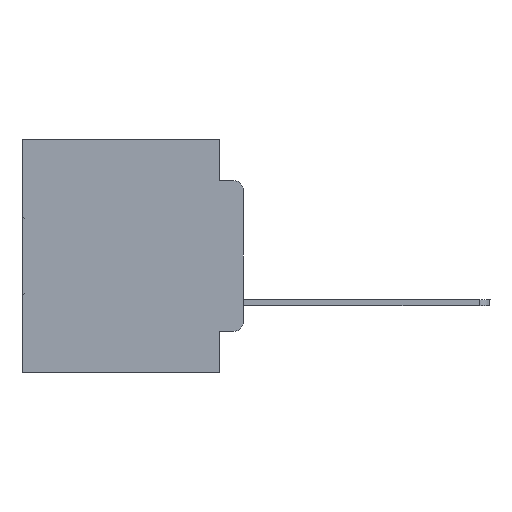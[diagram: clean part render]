
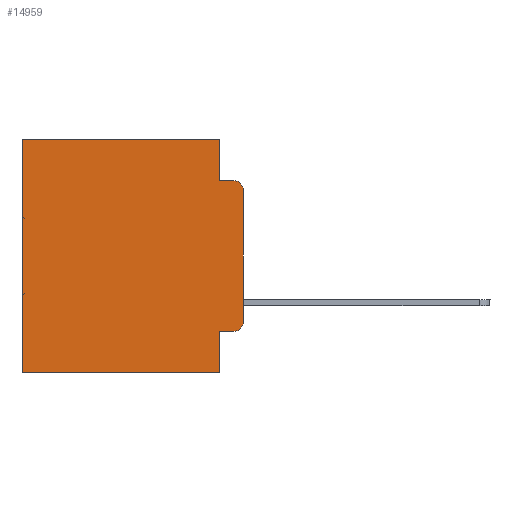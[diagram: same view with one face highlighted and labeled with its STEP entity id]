
A CAD part, left-side view. The second image highlights one B-rep face of the part: STEP entity #14959.
In plain terms, the highlighted planar face has unit normal (-1, 0, 0).
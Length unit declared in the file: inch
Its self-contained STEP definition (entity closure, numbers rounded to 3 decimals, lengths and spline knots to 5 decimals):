
#21 = DIRECTION ( 'NONE',  ( 0., 0., -1. ) ) ;
#1100 = VECTOR ( 'NONE', #27596, 39.37008 ) ;
#1137 = VECTOR ( 'NONE', #7769, 39.37008 ) ;
#1483 = ORIENTED_EDGE ( 'NONE', *, *, #3635, .T. ) ;
#2066 = CIRCLE ( 'NONE', #21026, 0.02 ) ;
#2542 = LINE ( 'NONE', #3341, #5845 ) ;
#3288 = VERTEX_POINT ( 'NONE', #8093 ) ;
#3341 = CARTESIAN_POINT ( 'NONE',  ( 0.298, 0., 0. ) ) ;
#3451 = DIRECTION ( 'NONE',  ( 0., 0., -1. ) ) ;
#3635 = EDGE_CURVE ( 'NONE', #31642, #13835, #26055, .T. ) ;
#4480 = ORIENTED_EDGE ( 'NONE', *, *, #25943, .T. ) ;
#4596 = CARTESIAN_POINT ( 'NONE',  ( 0.298, 0.02, -0.3915 ) ) ;
#4645 = EDGE_CURVE ( 'NONE', #8941, #17580, #16292, .T. ) ;
#5450 = VECTOR ( 'NONE', #10947, 39.37008 ) ;
#5484 = CIRCLE ( 'NONE', #14705, 0.02 ) ;
#5627 = LINE ( 'NONE', #23620, #17270 ) ;
#5845 = VECTOR ( 'NONE', #31802, 39.37008 ) ;
#5939 = VERTEX_POINT ( 'NONE', #24429 ) ;
#6153 = PLANE ( 'NONE',  #25862 ) ;
#6167 = VERTEX_POINT ( 'NONE', #28332 ) ;
#6237 = LINE ( 'NONE', #16592, #19477 ) ;
#7073 = CARTESIAN_POINT ( 'NONE',  ( 0.298, 0.051, -0.0885 ) ) ;
#7769 = DIRECTION ( 'NONE',  ( 0., -1., 0. ) ) ;
#7845 = DIRECTION ( 'NONE',  ( 0., 0., -1. ) ) ;
#7873 = ORIENTED_EDGE ( 'NONE', *, *, #23810, .F. ) ;
#8006 = LINE ( 'NONE', #10394, #9837 ) ;
#8093 = CARTESIAN_POINT ( 'NONE',  ( 0.298, 0.02, -0.4115 ) ) ;
#8941 = VERTEX_POINT ( 'NONE', #30897 ) ;
#9683 = ORIENTED_EDGE ( 'NONE', *, *, #16460, .F. ) ;
#9837 = VECTOR ( 'NONE', #7845, 39.37008 ) ;
#10394 = CARTESIAN_POINT ( 'NONE',  ( 0.298, 0.473, 0. ) ) ;
#10399 = DIRECTION ( 'NONE',  ( 0., 0., -1. ) ) ;
#10947 = DIRECTION ( 'NONE',  ( 0., 1., 0. ) ) ;
#12906 = DIRECTION ( 'NONE',  ( -1., 0., 0. ) ) ;
#13035 = ORIENTED_EDGE ( 'NONE', *, *, #18951, .T. ) ;
#13082 = VERTEX_POINT ( 'NONE', #28602 ) ;
#13779 = CARTESIAN_POINT ( 'NONE',  ( 0.298, 0.051, 0. ) ) ;
#13835 = VERTEX_POINT ( 'NONE', #32081 ) ;
#14062 = DIRECTION ( 'NONE',  ( 0., 1., 0. ) ) ;
#14705 = AXIS2_PLACEMENT_3D ( 'NONE', #4596, #27835, #31931 ) ;
#14959 = ADVANCED_FACE ( 'NONE', ( #29404 ), #6153, .F. ) ;
#15303 = CARTESIAN_POINT ( 'NONE',  ( 0.298, 0.02, -0.0885 ) ) ;
#15418 = LINE ( 'NONE', #22997, #1137 ) ;
#16176 = ORIENTED_EDGE ( 'NONE', *, *, #19793, .F. ) ;
#16292 = LINE ( 'NONE', #7073, #1100 ) ;
#16374 = CARTESIAN_POINT ( 'NONE',  ( 0.298, 0., 0. ) ) ;
#16460 = EDGE_CURVE ( 'NONE', #6167, #23488, #2542, .T. ) ;
#16592 = CARTESIAN_POINT ( 'NONE',  ( 0.298, 0., -0.5 ) ) ;
#16606 = ORIENTED_EDGE ( 'NONE', *, *, #19821, .F. ) ;
#16645 = VERTEX_POINT ( 'NONE', #32297 ) ;
#17270 = VECTOR ( 'NONE', #18208, 39.37008 ) ;
#17580 = VERTEX_POINT ( 'NONE', #15303 ) ;
#17601 = ORIENTED_EDGE ( 'NONE', *, *, #26426, .T. ) ;
#18208 = DIRECTION ( 'NONE',  ( 0., 0., -1. ) ) ;
#18595 = CARTESIAN_POINT ( 'NONE',  ( 0.298, 0.051, 0. ) ) ;
#18951 = EDGE_CURVE ( 'NONE', #6167, #17580, #2066, .T. ) ;
#19477 = VECTOR ( 'NONE', #14062, 39.37008 ) ;
#19793 = EDGE_CURVE ( 'NONE', #31642, #8941, #5627, .T. ) ;
#19821 = EDGE_CURVE ( 'NONE', #5939, #16645, #29206, .T. ) ;
#21026 = AXIS2_PLACEMENT_3D ( 'NONE', #31190, #12906, #21 ) ;
#22997 = CARTESIAN_POINT ( 'NONE',  ( 0.298, 0.051, -0.4115 ) ) ;
#23488 = VERTEX_POINT ( 'NONE', #33060 ) ;
#23620 = CARTESIAN_POINT ( 'NONE',  ( 0.298, 0.051, 0. ) ) ;
#23810 = EDGE_CURVE ( 'NONE', #16645, #13082, #6237, .T. ) ;
#24429 = CARTESIAN_POINT ( 'NONE',  ( 0.298, 0.051, -0.4115 ) ) ;
#25862 = AXIS2_PLACEMENT_3D ( 'NONE', #26695, #32086, #3451 ) ;
#25943 = EDGE_CURVE ( 'NONE', #3288, #23488, #5484, .T. ) ;
#26055 = LINE ( 'NONE', #16374, #5450 ) ;
#26419 = ORIENTED_EDGE ( 'NONE', *, *, #4645, .F. ) ;
#26426 = EDGE_CURVE ( 'NONE', #5939, #3288, #15418, .T. ) ;
#26695 = CARTESIAN_POINT ( 'NONE',  ( 0.298, 0., 0. ) ) ;
#27596 = DIRECTION ( 'NONE',  ( 0., -1., 0. ) ) ;
#27606 = VECTOR ( 'NONE', #10399, 39.37008 ) ;
#27835 = DIRECTION ( 'NONE',  ( -1., 0., 0. ) ) ;
#28332 = CARTESIAN_POINT ( 'NONE',  ( 0.298, 0., -0.1085 ) ) ;
#28602 = CARTESIAN_POINT ( 'NONE',  ( 0.298, 0.473, -0.5 ) ) ;
#29206 = LINE ( 'NONE', #13779, #27606 ) ;
#29404 = FACE_OUTER_BOUND ( 'NONE', #31677, .T. ) ;
#30897 = CARTESIAN_POINT ( 'NONE',  ( 0.298, 0.051, -0.0885 ) ) ;
#30962 = EDGE_CURVE ( 'NONE', #13835, #13082, #8006, .T. ) ;
#31190 = CARTESIAN_POINT ( 'NONE',  ( 0.298, 0.02, -0.1085 ) ) ;
#31517 = ORIENTED_EDGE ( 'NONE', *, *, #30962, .T. ) ;
#31642 = VERTEX_POINT ( 'NONE', #18595 ) ;
#31677 = EDGE_LOOP ( 'NONE', ( #9683, #13035, #26419, #16176, #1483, #31517, #7873, #16606, #17601, #4480 ) ) ;
#31802 = DIRECTION ( 'NONE',  ( 0., 0., -1. ) ) ;
#31931 = DIRECTION ( 'NONE',  ( 0., 0., -1. ) ) ;
#32081 = CARTESIAN_POINT ( 'NONE',  ( 0.298, 0.473, 0. ) ) ;
#32086 = DIRECTION ( 'NONE',  ( 1., 0., 0. ) ) ;
#32297 = CARTESIAN_POINT ( 'NONE',  ( 0.298, 0.051, -0.5 ) ) ;
#33060 = CARTESIAN_POINT ( 'NONE',  ( 0.298, 0., -0.3915 ) ) ;
